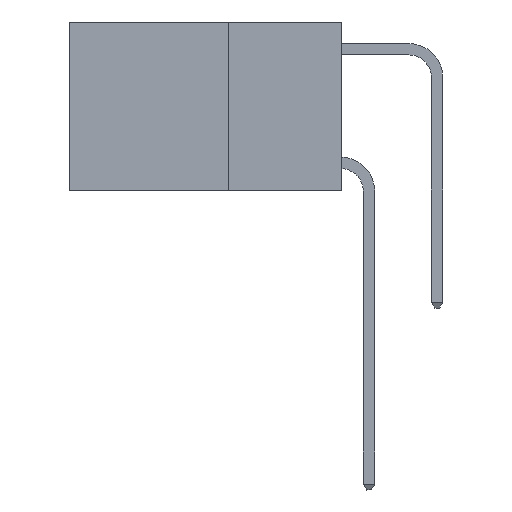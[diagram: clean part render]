
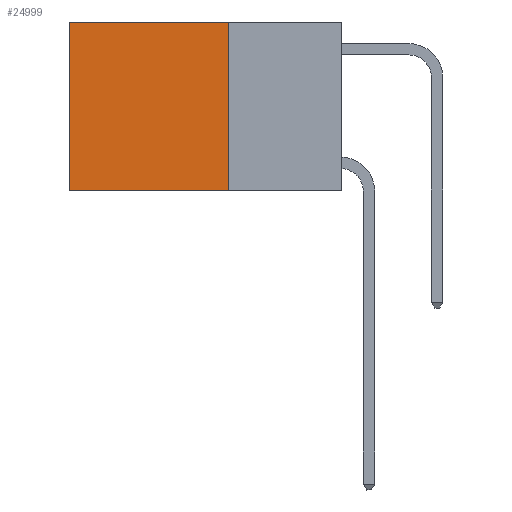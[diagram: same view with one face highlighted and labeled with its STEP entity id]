
A CAD part, left-side view. The second image highlights one B-rep face of the part: STEP entity #24999.
In plain terms, the highlighted planar face has unit normal (-1, 0, 0).
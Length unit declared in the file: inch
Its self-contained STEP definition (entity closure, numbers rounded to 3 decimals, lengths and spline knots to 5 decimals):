
#1071 = CARTESIAN_POINT ( 'NONE',  ( 0.2625, 0.6, 0. ) ) ;
#1317 = CARTESIAN_POINT ( 'NONE',  ( 0.2625, 0.25, -0.37 ) ) ;
#1432 = LINE ( 'NONE', #7929, #13169 ) ;
#1737 = CARTESIAN_POINT ( 'NONE',  ( 0.2625, 0.25, 0. ) ) ;
#2697 = LINE ( 'NONE', #29569, #12967 ) ;
#2732 = EDGE_CURVE ( 'NONE', #17981, #5481, #2697, .T. ) ;
#3020 = VERTEX_POINT ( 'NONE', #23613 ) ;
#4417 = ORIENTED_EDGE ( 'NONE', *, *, #23796, .T. ) ;
#5481 = VERTEX_POINT ( 'NONE', #1071 ) ;
#5745 = LINE ( 'NONE', #22571, #11268 ) ;
#5754 = FACE_OUTER_BOUND ( 'NONE', #19263, .T. ) ;
#7929 = CARTESIAN_POINT ( 'NONE',  ( 0.2625, 0.6, 0. ) ) ;
#9419 = VERTEX_POINT ( 'NONE', #18550 ) ;
#9614 = PLANE ( 'NONE',  #28668 ) ;
#10821 = ORIENTED_EDGE ( 'NONE', *, *, #15220, .F. ) ;
#11268 = VECTOR ( 'NONE', #24936, 39.37008 ) ;
#11679 = LINE ( 'NONE', #1317, #23445 ) ;
#11964 = CARTESIAN_POINT ( 'NONE',  ( 0.2625, 0.25, 0. ) ) ;
#12967 = VECTOR ( 'NONE', #15501, 39.37008 ) ;
#13169 = VECTOR ( 'NONE', #21990, 39.37008 ) ;
#14299 = DIRECTION ( 'NONE',  ( 0., 0., -1. ) ) ;
#15220 = EDGE_CURVE ( 'NONE', #17981, #3020, #5745, .T. ) ;
#15501 = DIRECTION ( 'NONE',  ( 0., 1., 0. ) ) ;
#17981 = VERTEX_POINT ( 'NONE', #1737 ) ;
#18550 = CARTESIAN_POINT ( 'NONE',  ( 0.2625, 0.6, -0.37 ) ) ;
#19263 = EDGE_LOOP ( 'NONE', ( #4417, #22464, #10821, #20021 ) ) ;
#20021 = ORIENTED_EDGE ( 'NONE', *, *, #2732, .T. ) ;
#21990 = DIRECTION ( 'NONE',  ( 0., 0., -1. ) ) ;
#22464 = ORIENTED_EDGE ( 'NONE', *, *, #27994, .F. ) ;
#22571 = CARTESIAN_POINT ( 'NONE',  ( 0.2625, 0.25, 0. ) ) ;
#23445 = VECTOR ( 'NONE', #24720, 39.37008 ) ;
#23613 = CARTESIAN_POINT ( 'NONE',  ( 0.2625, 0.25, -0.37 ) ) ;
#23796 = EDGE_CURVE ( 'NONE', #5481, #9419, #1432, .T. ) ;
#24720 = DIRECTION ( 'NONE',  ( 0., 1., 0. ) ) ;
#24936 = DIRECTION ( 'NONE',  ( 0., 0., -1. ) ) ;
#24999 = ADVANCED_FACE ( 'NONE', ( #5754 ), #9614, .F. ) ;
#27994 = EDGE_CURVE ( 'NONE', #3020, #9419, #11679, .T. ) ;
#28382 = DIRECTION ( 'NONE',  ( 1., 0., 0. ) ) ;
#28668 = AXIS2_PLACEMENT_3D ( 'NONE', #11964, #28382, #14299 ) ;
#29569 = CARTESIAN_POINT ( 'NONE',  ( 0.2625, 0.25, 0. ) ) ;
